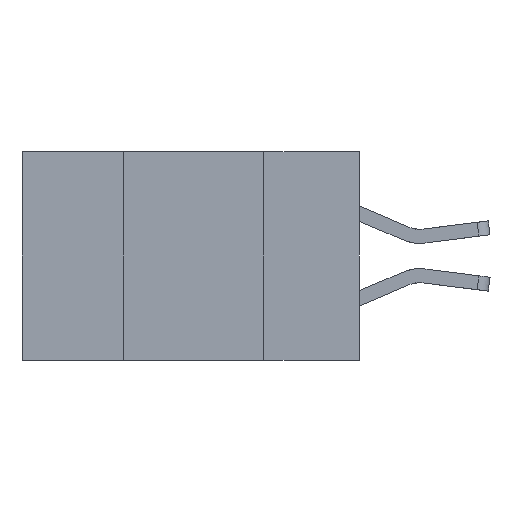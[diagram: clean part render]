
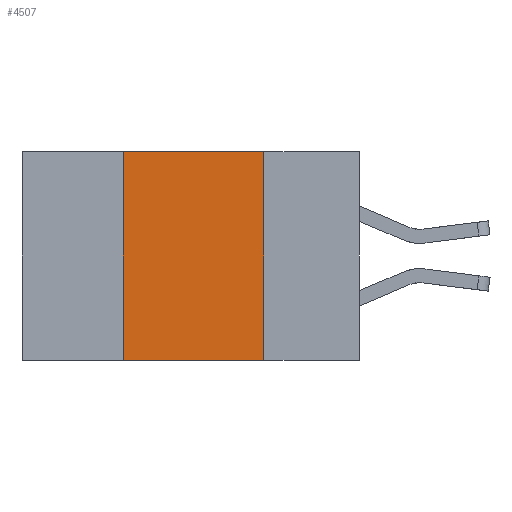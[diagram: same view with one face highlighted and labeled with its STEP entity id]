
A CAD part, left-side view. The second image highlights one B-rep face of the part: STEP entity #4507.
In plain terms, the highlighted planar face has unit normal (-1, 0, 0).
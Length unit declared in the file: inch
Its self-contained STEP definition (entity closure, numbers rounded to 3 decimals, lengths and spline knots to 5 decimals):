
#643 = VECTOR ( 'NONE', #2959, 39.37008 ) ;
#720 = AXIS2_PLACEMENT_3D ( 'NONE', #11627, #3067, #11761 ) ;
#1527 = CARTESIAN_POINT ( 'NONE',  ( 0., 0.42, 0. ) ) ;
#1765 = CARTESIAN_POINT ( 'NONE',  ( 0., 0.6, 0. ) ) ;
#1818 = LINE ( 'NONE', #9372, #643 ) ;
#2213 = EDGE_CURVE ( 'NONE', #3159, #4205, #9738, .T. ) ;
#2520 = ORIENTED_EDGE ( 'NONE', *, *, #6239, .F. ) ;
#2959 = DIRECTION ( 'NONE',  ( 0., 0., -1. ) ) ;
#3067 = DIRECTION ( 'NONE',  ( 1., 0., 0. ) ) ;
#3159 = VERTEX_POINT ( 'NONE', #11260 ) ;
#3690 = DIRECTION ( 'NONE',  ( 0., 0., 1. ) ) ;
#4205 = VERTEX_POINT ( 'NONE', #6647 ) ;
#4500 = ORIENTED_EDGE ( 'NONE', *, *, #9685, .F. ) ;
#4507 = ADVANCED_FACE ( 'NONE', ( #13536 ), #9469, .F. ) ;
#4693 = VECTOR ( 'NONE', #3690, 39.37008 ) ;
#5360 = LINE ( 'NONE', #11097, #4693 ) ;
#5488 = ORIENTED_EDGE ( 'NONE', *, *, #11172, .F. ) ;
#6239 = EDGE_CURVE ( 'NONE', #6351, #4205, #1818, .T. ) ;
#6351 = VERTEX_POINT ( 'NONE', #7951 ) ;
#6647 = CARTESIAN_POINT ( 'NONE',  ( 0., 0.17, -0.37 ) ) ;
#6662 = DIRECTION ( 'NONE',  ( 0., -1., 0. ) ) ;
#7951 = CARTESIAN_POINT ( 'NONE',  ( 0., 0.17, 0. ) ) ;
#8278 = EDGE_LOOP ( 'NONE', ( #2520, #4500, #5488, #11734 ) ) ;
#9209 = VECTOR ( 'NONE', #9237, 39.37008 ) ;
#9221 = LINE ( 'NONE', #1765, #9209 ) ;
#9237 = DIRECTION ( 'NONE',  ( 0., -1., 0. ) ) ;
#9372 = CARTESIAN_POINT ( 'NONE',  ( 0., 0.17, 0. ) ) ;
#9469 = PLANE ( 'NONE',  #720 ) ;
#9599 = VERTEX_POINT ( 'NONE', #1527 ) ;
#9685 = EDGE_CURVE ( 'NONE', #9599, #6351, #9221, .T. ) ;
#9738 = LINE ( 'NONE', #11958, #10383 ) ;
#10383 = VECTOR ( 'NONE', #6662, 39.37008 ) ;
#11097 = CARTESIAN_POINT ( 'NONE',  ( 0., 0.42, 0. ) ) ;
#11172 = EDGE_CURVE ( 'NONE', #3159, #9599, #5360, .T. ) ;
#11260 = CARTESIAN_POINT ( 'NONE',  ( 0., 0.42, -0.37 ) ) ;
#11627 = CARTESIAN_POINT ( 'NONE',  ( 0., 0.6, 0. ) ) ;
#11734 = ORIENTED_EDGE ( 'NONE', *, *, #2213, .T. ) ;
#11761 = DIRECTION ( 'NONE',  ( 0., 0., -1. ) ) ;
#11958 = CARTESIAN_POINT ( 'NONE',  ( 0., 0.6, -0.37 ) ) ;
#13536 = FACE_OUTER_BOUND ( 'NONE', #8278, .T. ) ;
